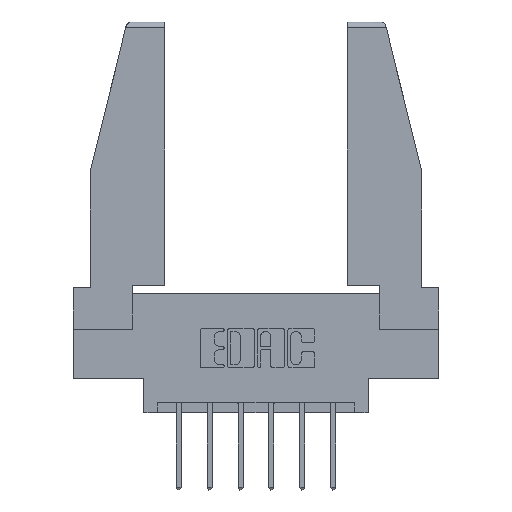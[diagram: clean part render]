
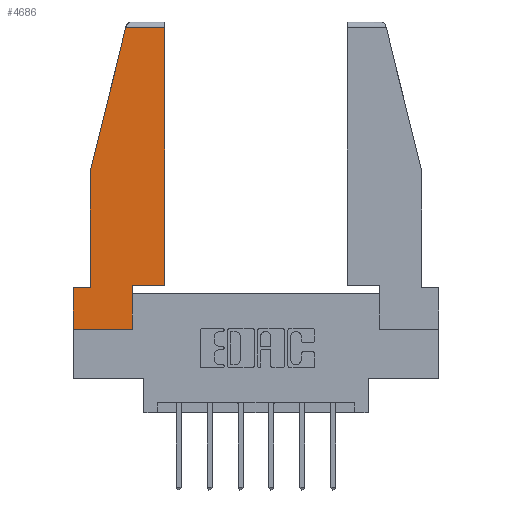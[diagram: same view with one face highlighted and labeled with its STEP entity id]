
A CAD part, top view. The second image highlights one B-rep face of the part: STEP entity #4686.
In plain terms, the highlighted planar face has unit normal (0, 0, 1).
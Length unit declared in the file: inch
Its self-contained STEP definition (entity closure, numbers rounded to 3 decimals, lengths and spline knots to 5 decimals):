
#7 = VECTOR ( 'NONE', #7985, 39.37008 ) ;
#13 = CARTESIAN_POINT ( 'NONE',  ( 0.461, 0.223, 0. ) ) ;
#59 = CARTESIAN_POINT ( 'NONE',  ( 0.086, 0.8, 0. ) ) ;
#66 = FACE_OUTER_BOUND ( 'NONE', #8221, .T. ) ;
#75 = VERTEX_POINT ( 'NONE', #1227 ) ;
#269 = PLANE ( 'NONE',  #4945 ) ;
#385 = DIRECTION ( 'NONE',  ( 0., 0., 1. ) ) ;
#724 = CARTESIAN_POINT ( 'NONE',  ( 0., 0.21, 0. ) ) ;
#817 = VERTEX_POINT ( 'NONE', #10622 ) ;
#874 = VECTOR ( 'NONE', #7439, 39.37008 ) ;
#1034 = EDGE_CURVE ( 'NONE', #4143, #5152, #7909, .T. ) ;
#1209 = CARTESIAN_POINT ( 'NONE',  ( 0.297, 0., 0. ) ) ;
#1216 = LINE ( 'NONE', #9115, #3646 ) ;
#1227 = CARTESIAN_POINT ( 'NONE',  ( 0.297, 0., 0. ) ) ;
#1491 = VECTOR ( 'NONE', #2317, 39.37008 ) ;
#1593 = CARTESIAN_POINT ( 'NONE',  ( 0.297, 0.223, 0. ) ) ;
#1762 = LINE ( 'NONE', #1593, #7 ) ;
#2127 = CARTESIAN_POINT ( 'NONE',  ( 0., 0.21, 0. ) ) ;
#2168 = DIRECTION ( 'NONE',  ( -1., 0., 0. ) ) ;
#2210 = EDGE_CURVE ( 'NONE', #6218, #4143, #6019, .T. ) ;
#2317 = DIRECTION ( 'NONE',  ( -0.239, -0.971, 0. ) ) ;
#3036 = DIRECTION ( 'NONE',  ( -1., 0., 0. ) ) ;
#3174 = DIRECTION ( 'NONE',  ( 0., -1., 0. ) ) ;
#3235 = CARTESIAN_POINT ( 'NONE',  ( 0.271, 1.55, 0. ) ) ;
#3268 = EDGE_CURVE ( 'NONE', #4944, #11488, #7608, .T. ) ;
#3340 = LINE ( 'NONE', #3235, #1491 ) ;
#3404 = CARTESIAN_POINT ( 'NONE',  ( 0., 1.52, 0. ) ) ;
#3514 = ORIENTED_EDGE ( 'NONE', *, *, #3268, .T. ) ;
#3646 = VECTOR ( 'NONE', #10067, 39.37008 ) ;
#3907 = LINE ( 'NONE', #1209, #11679 ) ;
#4143 = VERTEX_POINT ( 'NONE', #7266 ) ;
#4608 = CARTESIAN_POINT ( 'NONE',  ( 0., 0., 0. ) ) ;
#4686 = ADVANCED_FACE ( 'NONE', ( #66 ), #269, .T. ) ;
#4944 = VERTEX_POINT ( 'NONE', #724 ) ;
#4945 = AXIS2_PLACEMENT_3D ( 'NONE', #9545, #385, #9507 ) ;
#5077 = ORIENTED_EDGE ( 'NONE', *, *, #1034, .T. ) ;
#5152 = VERTEX_POINT ( 'NONE', #11925 ) ;
#5412 = ORIENTED_EDGE ( 'NONE', *, *, #8853, .T. ) ;
#5457 = VECTOR ( 'NONE', #2168, 39.37008 ) ;
#5767 = ORIENTED_EDGE ( 'NONE', *, *, #11888, .T. ) ;
#5788 = ORIENTED_EDGE ( 'NONE', *, *, #11823, .T. ) ;
#6019 = LINE ( 'NONE', #9883, #8327 ) ;
#6217 = DIRECTION ( 'NONE',  ( 0., 1., 0. ) ) ;
#6218 = VERTEX_POINT ( 'NONE', #13 ) ;
#6357 = VECTOR ( 'NONE', #3036, 39.37008 ) ;
#7008 = EDGE_CURVE ( 'NONE', #8800, #9589, #1216, .T. ) ;
#7266 = CARTESIAN_POINT ( 'NONE',  ( 0.461, 1.52, 0. ) ) ;
#7439 = DIRECTION ( 'NONE',  ( 1., 0., 0. ) ) ;
#7608 = LINE ( 'NONE', #2127, #10489 ) ;
#7682 = ORIENTED_EDGE ( 'NONE', *, *, #11559, .T. ) ;
#7909 = LINE ( 'NONE', #3404, #5457 ) ;
#7985 = DIRECTION ( 'NONE',  ( 1., 0., 0. ) ) ;
#8024 = ORIENTED_EDGE ( 'NONE', *, *, #7008, .T. ) ;
#8221 = EDGE_LOOP ( 'NONE', ( #11370, #5077, #5767, #8024, #11042, #3514, #5412, #5788, #7682 ) ) ;
#8327 = VECTOR ( 'NONE', #6217, 39.37008 ) ;
#8554 = CARTESIAN_POINT ( 'NONE',  ( 0., 0.21, 0. ) ) ;
#8800 = VERTEX_POINT ( 'NONE', #59 ) ;
#8819 = LINE ( 'NONE', #8554, #6357 ) ;
#8853 = EDGE_CURVE ( 'NONE', #11488, #75, #10087, .T. ) ;
#9115 = CARTESIAN_POINT ( 'NONE',  ( 0.086, 0.8, 0. ) ) ;
#9507 = DIRECTION ( 'NONE',  ( 1., 0., 0. ) ) ;
#9545 = CARTESIAN_POINT ( 'NONE',  ( 0., 0., 0. ) ) ;
#9589 = VERTEX_POINT ( 'NONE', #10174 ) ;
#9883 = CARTESIAN_POINT ( 'NONE',  ( 0.461, 0.223, 0. ) ) ;
#10067 = DIRECTION ( 'NONE',  ( 0., -1., 0. ) ) ;
#10087 = LINE ( 'NONE', #4608, #874 ) ;
#10174 = CARTESIAN_POINT ( 'NONE',  ( 0.086, 0.21, 0. ) ) ;
#10489 = VECTOR ( 'NONE', #3174, 39.37008 ) ;
#10622 = CARTESIAN_POINT ( 'NONE',  ( 0.297, 0.223, 0. ) ) ;
#11042 = ORIENTED_EDGE ( 'NONE', *, *, #11203, .T. ) ;
#11203 = EDGE_CURVE ( 'NONE', #9589, #4944, #8819, .T. ) ;
#11293 = DIRECTION ( 'NONE',  ( 0., 1., 0. ) ) ;
#11370 = ORIENTED_EDGE ( 'NONE', *, *, #2210, .T. ) ;
#11488 = VERTEX_POINT ( 'NONE', #11808 ) ;
#11559 = EDGE_CURVE ( 'NONE', #817, #6218, #1762, .T. ) ;
#11679 = VECTOR ( 'NONE', #11293, 39.37008 ) ;
#11808 = CARTESIAN_POINT ( 'NONE',  ( 0., 0., 0. ) ) ;
#11823 = EDGE_CURVE ( 'NONE', #75, #817, #3907, .T. ) ;
#11888 = EDGE_CURVE ( 'NONE', #5152, #8800, #3340, .T. ) ;
#11925 = CARTESIAN_POINT ( 'NONE',  ( 0.2636, 1.52, 0. ) ) ;
